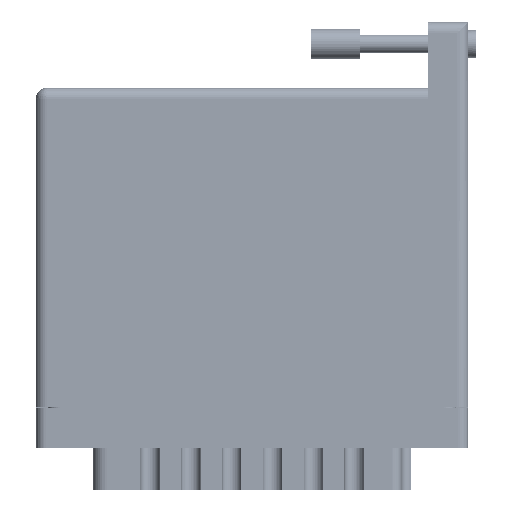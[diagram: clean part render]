
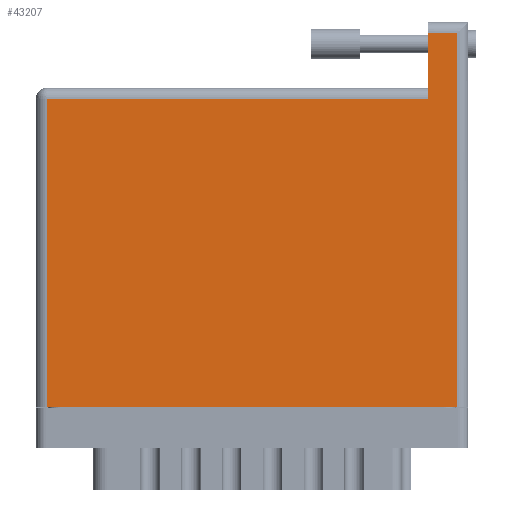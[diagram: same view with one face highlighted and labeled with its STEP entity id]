
A CAD part, front view. The second image highlights one B-rep face of the part: STEP entity #43207.
In plain terms, the highlighted face is planar.
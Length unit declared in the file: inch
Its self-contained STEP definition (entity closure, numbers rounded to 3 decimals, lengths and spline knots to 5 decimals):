
#285 = ORIENTED_EDGE ( 'NONE', *, *, #45160, .T. ) ;
#1350 = EDGE_CURVE ( 'NONE', #3759, #40757, #73760, .T. ) ;
#1843 = CARTESIAN_POINT ( 'NONE',  ( 0., 2.03, 0. ) ) ;
#3759 = VERTEX_POINT ( 'NONE', #63089 ) ;
#7905 = CARTESIAN_POINT ( 'NONE',  ( 0., 0., 0. ) ) ;
#9177 = LINE ( 'NONE', #85675, #31302 ) ;
#16264 = LINE ( 'NONE', #7905, #76879 ) ;
#16441 = DIRECTION ( 'NONE',  ( -1., 0., 0. ) ) ;
#24941 = FACE_OUTER_BOUND ( 'NONE', #45067, .T. ) ;
#25432 = LINE ( 'NONE', #32137, #83673 ) ;
#28226 = CARTESIAN_POINT ( 'NONE',  ( 0.07, 0., 0. ) ) ;
#30890 = CARTESIAN_POINT ( 'NONE',  ( 0., 2.38, 0. ) ) ;
#31302 = VECTOR ( 'NONE', #70401, 39.37008 ) ;
#32137 = CARTESIAN_POINT ( 'NONE',  ( 2.685, 2.45, 0. ) ) ;
#34113 = VECTOR ( 'NONE', #83007, 39.37008 ) ;
#35849 = VECTOR ( 'NONE', #88141, 39.37008 ) ;
#36066 = ORIENTED_EDGE ( 'NONE', *, *, #49883, .T. ) ;
#37975 = PLANE ( 'NONE',  #77317 ) ;
#40757 = VERTEX_POINT ( 'NONE', #59059 ) ;
#43207 = ADVANCED_FACE ( 'NONE', ( #24941 ), #37975, .F. ) ;
#45067 = EDGE_LOOP ( 'NONE', ( #80699, #36066, #80686, #285, #63667, #67107 ) ) ;
#45160 = EDGE_CURVE ( 'NONE', #49227, #90186, #16264, .T. ) ;
#47268 = CARTESIAN_POINT ( 'NONE',  ( 0.07, 0., 0. ) ) ;
#49211 = VECTOR ( 'NONE', #92041, 39.37008 ) ;
#49227 = VERTEX_POINT ( 'NONE', #47268 ) ;
#49883 = EDGE_CURVE ( 'NONE', #72220, #92088, #53888, .T. ) ;
#53641 = DIRECTION ( 'NONE',  ( 0., 1., 0. ) ) ;
#53888 = LINE ( 'NONE', #77475, #49211 ) ;
#57552 = EDGE_CURVE ( 'NONE', #92088, #49227, #95212, .T. ) ;
#59059 = CARTESIAN_POINT ( 'NONE',  ( 2.499, 2.38, 0. ) ) ;
#60633 = DIRECTION ( 'NONE',  ( 1., 0., 0. ) ) ;
#63089 = CARTESIAN_POINT ( 'NONE',  ( 2.685, 2.38, 0. ) ) ;
#63667 = ORIENTED_EDGE ( 'NONE', *, *, #68989, .T. ) ;
#66148 = CARTESIAN_POINT ( 'NONE',  ( 2.685, 0., 0. ) ) ;
#67107 = ORIENTED_EDGE ( 'NONE', *, *, #1350, .T. ) ;
#68989 = EDGE_CURVE ( 'NONE', #90186, #3759, #25432, .T. ) ;
#70401 = DIRECTION ( 'NONE',  ( 0., -1., 0. ) ) ;
#72220 = VERTEX_POINT ( 'NONE', #83940 ) ;
#73316 = CARTESIAN_POINT ( 'NONE',  ( 0.07, 1.96, 0. ) ) ;
#73760 = LINE ( 'NONE', #30890, #34113 ) ;
#76879 = VECTOR ( 'NONE', #60633, 39.37008 ) ;
#77317 = AXIS2_PLACEMENT_3D ( 'NONE', #1843, #82904, #16441 ) ;
#77475 = CARTESIAN_POINT ( 'NONE',  ( 0., 1.96, 0. ) ) ;
#80686 = ORIENTED_EDGE ( 'NONE', *, *, #57552, .T. ) ;
#80699 = ORIENTED_EDGE ( 'NONE', *, *, #94584, .T. ) ;
#82904 = DIRECTION ( 'NONE',  ( 0., 0., -1. ) ) ;
#83007 = DIRECTION ( 'NONE',  ( -1., 0., 0. ) ) ;
#83673 = VECTOR ( 'NONE', #53641, 39.37008 ) ;
#83940 = CARTESIAN_POINT ( 'NONE',  ( 2.499, 1.96, 0. ) ) ;
#85675 = CARTESIAN_POINT ( 'NONE',  ( 2.499, 2.45, 0. ) ) ;
#88141 = DIRECTION ( 'NONE',  ( 0., -1., 0. ) ) ;
#90186 = VERTEX_POINT ( 'NONE', #66148 ) ;
#92041 = DIRECTION ( 'NONE',  ( -1., 0., 0. ) ) ;
#92088 = VERTEX_POINT ( 'NONE', #73316 ) ;
#94584 = EDGE_CURVE ( 'NONE', #40757, #72220, #9177, .T. ) ;
#95212 = LINE ( 'NONE', #28226, #35849 ) ;
